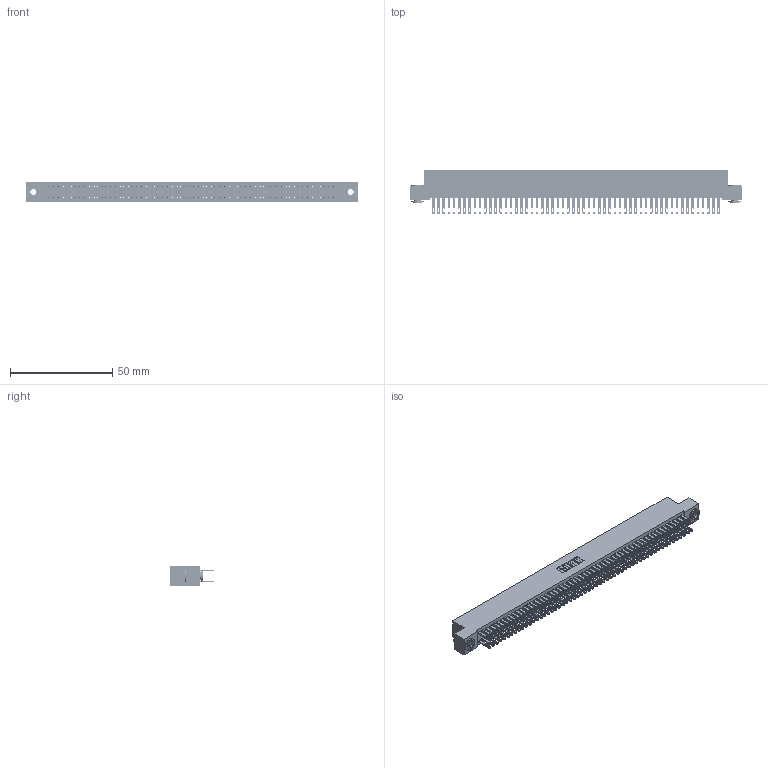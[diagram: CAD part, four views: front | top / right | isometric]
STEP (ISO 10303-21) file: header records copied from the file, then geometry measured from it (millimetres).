
FILE_DESCRIPTION (( 'STEP AP203' ), '1' );
FILE_NAME ('892-112-500-203.STEP', '2020-09-21T21:59:59', ( '' ), ( '' ), 'SwSTEP 2.0', 'SolidWorks 2020', '' );
FILE_SCHEMA (( 'CONFIG_CONTROL_DESIGN' ));
Length unit declared in the file: inch
Products named in the file (4): 342-250-002_345-250-002-102; 345-292-001_345-293-100; 892-112-500-203; 842 Part_.156 TH
Assembly tree (115 placements, depth 2):
  892-112-500-203
    842 Part_.156 TH
    345-292-001_345-293-100  x112
    342-250-002_345-250-002-102  x2
Bounding box: 162.56 x 21.85 x 9.4 mm (x, y, z)
Volume: 15037.3 mm3; surface area: 26108.4 mm2
Topology: 115 solids, 115 shells, 5524 faces, 16839 edges, 11222 vertices
Faces by surface type: plane 3436, cylinder 2080, cone 8
Entity records: 34664 total; most frequent: CARTESIAN_POINT 5701, ORIENTED_EDGE 5630, DIRECTION 4881, EDGE_CURVE 2815, LINE 2659, VECTOR 2659, VERTEX_POINT 1874, AXIS2_PLACEMENT_3D 1111
